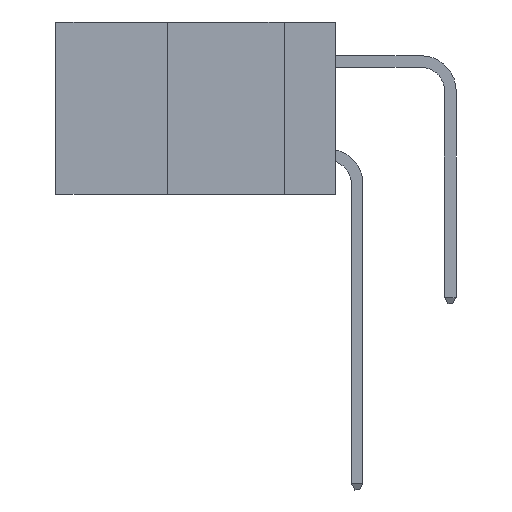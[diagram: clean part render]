
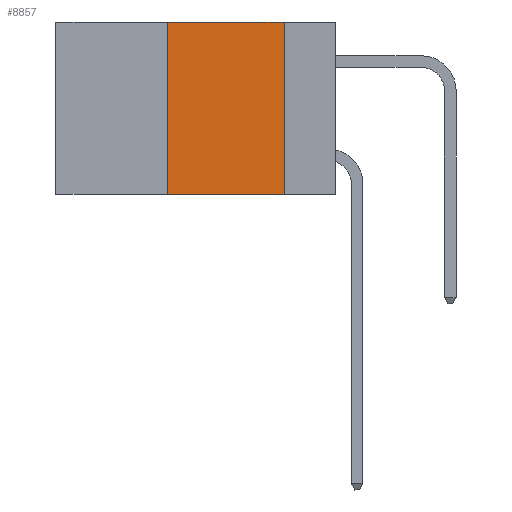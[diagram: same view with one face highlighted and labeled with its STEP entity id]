
A CAD part, left-side view. The second image highlights one B-rep face of the part: STEP entity #8857.
In plain terms, the highlighted planar face has unit normal (-1, 0, 0).
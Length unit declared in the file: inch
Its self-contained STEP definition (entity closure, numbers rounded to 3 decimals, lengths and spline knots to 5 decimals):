
#326 = DIRECTION ( 'NONE',  ( 1., 0., 0. ) ) ;
#533 = LINE ( 'NONE', #8390, #8734 ) ;
#1028 = EDGE_CURVE ( 'NONE', #10397, #7891, #533, .T. ) ;
#1589 = VECTOR ( 'NONE', #9934, 39.37008 ) ;
#1684 = VERTEX_POINT ( 'NONE', #6394 ) ;
#1728 = FACE_OUTER_BOUND ( 'NONE', #4316, .T. ) ;
#2233 = CARTESIAN_POINT ( 'NONE',  ( 0., 0.6, -0.37 ) ) ;
#2375 = ORIENTED_EDGE ( 'NONE', *, *, #9887, .F. ) ;
#2549 = VERTEX_POINT ( 'NONE', #10951 ) ;
#3224 = CARTESIAN_POINT ( 'NONE',  ( 0., 0.36, -0.37 ) ) ;
#3395 = DIRECTION ( 'NONE',  ( 0., 0., -1. ) ) ;
#4075 = EDGE_CURVE ( 'NONE', #10397, #2549, #4473, .T. ) ;
#4316 = EDGE_LOOP ( 'NONE', ( #2375, #8601, #9497, #5412 ) ) ;
#4473 = LINE ( 'NONE', #2233, #1589 ) ;
#5412 = ORIENTED_EDGE ( 'NONE', *, *, #4075, .T. ) ;
#6394 = CARTESIAN_POINT ( 'NONE',  ( 0., 0.11, 0. ) ) ;
#6874 = CARTESIAN_POINT ( 'NONE',  ( 0., 0.6, 0. ) ) ;
#7071 = EDGE_CURVE ( 'NONE', #7891, #1684, #10650, .T. ) ;
#7845 = VECTOR ( 'NONE', #3395, 39.37008 ) ;
#7883 = DIRECTION ( 'NONE',  ( 0., 0., -1. ) ) ;
#7891 = VERTEX_POINT ( 'NONE', #10162 ) ;
#8089 = VECTOR ( 'NONE', #11689, 39.37008 ) ;
#8390 = CARTESIAN_POINT ( 'NONE',  ( 0., 0.36, 0. ) ) ;
#8601 = ORIENTED_EDGE ( 'NONE', *, *, #7071, .F. ) ;
#8734 = VECTOR ( 'NONE', #10222, 39.37008 ) ;
#8857 = ADVANCED_FACE ( 'NONE', ( #1728 ), #11647, .F. ) ;
#9497 = ORIENTED_EDGE ( 'NONE', *, *, #1028, .F. ) ;
#9887 = EDGE_CURVE ( 'NONE', #1684, #2549, #10413, .T. ) ;
#9934 = DIRECTION ( 'NONE',  ( 0., -1., 0. ) ) ;
#10162 = CARTESIAN_POINT ( 'NONE',  ( 0., 0.36, 0. ) ) ;
#10222 = DIRECTION ( 'NONE',  ( 0., 0., 1. ) ) ;
#10397 = VERTEX_POINT ( 'NONE', #3224 ) ;
#10413 = LINE ( 'NONE', #10474, #7845 ) ;
#10474 = CARTESIAN_POINT ( 'NONE',  ( 0., 0.11, 0. ) ) ;
#10650 = LINE ( 'NONE', #10787, #8089 ) ;
#10684 = AXIS2_PLACEMENT_3D ( 'NONE', #6874, #326, #7883 ) ;
#10787 = CARTESIAN_POINT ( 'NONE',  ( 0., 0.6, 0. ) ) ;
#10951 = CARTESIAN_POINT ( 'NONE',  ( 0., 0.11, -0.37 ) ) ;
#11647 = PLANE ( 'NONE',  #10684 ) ;
#11689 = DIRECTION ( 'NONE',  ( 0., -1., 0. ) ) ;
